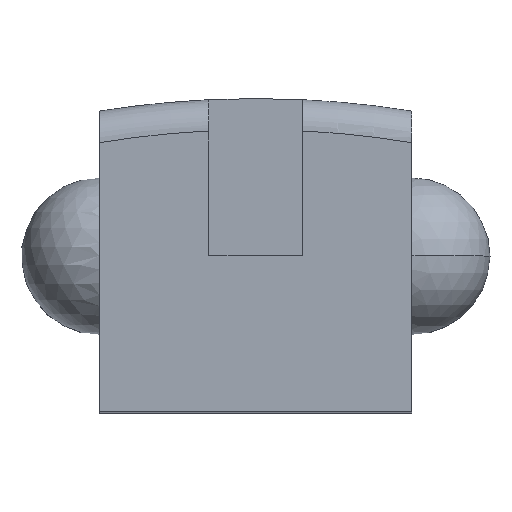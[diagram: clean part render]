
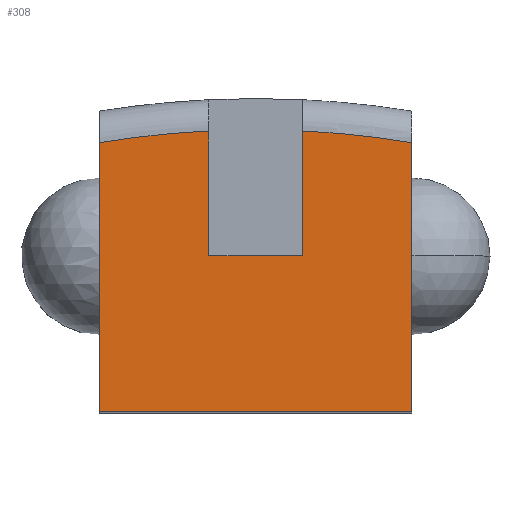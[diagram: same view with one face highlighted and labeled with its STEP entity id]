
A CAD part, top view. The second image highlights one B-rep face of the part: STEP entity #308.
In plain terms, the highlighted planar face has unit normal (0, 0, 1).
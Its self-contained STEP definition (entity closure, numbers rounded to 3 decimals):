
#2 = DIRECTION ( 'NONE',  ( 0., -1., 0. ) ) ;
#4 = CARTESIAN_POINT ( 'NONE',  ( 6.5, -1.25, 12.5 ) ) ;
#25 = CARTESIAN_POINT ( 'NONE',  ( 6.5, -1.25, 12.5 ) ) ;
#34 = DIRECTION ( 'NONE',  ( 0., 0., 1. ) ) ;
#44 = CARTESIAN_POINT ( 'NONE',  ( 3.5, -1.25, 12.5 ) ) ;
#46 = DIRECTION ( 'NONE',  ( 0., 1., 0. ) ) ;
#47 = DIRECTION ( 'NONE',  ( 0., -1., 0. ) ) ;
#55 = DIRECTION ( 'NONE',  ( -1., 0., 0. ) ) ;
#70 = DIRECTION ( 'NONE',  ( 0., 0., 1. ) ) ;
#90 = CARTESIAN_POINT ( 'NONE',  ( 6.5, 2.747, 12.5 ) ) ;
#99 = CARTESIAN_POINT ( 'NONE',  ( 10., -6.25, 12.5 ) ) ;
#117 = CARTESIAN_POINT ( 'NONE',  ( 0., -6.25, 12.5 ) ) ;
#131 = CARTESIAN_POINT ( 'NONE',  ( 10., -6.25, 12.5 ) ) ;
#154 = CARTESIAN_POINT ( 'NONE',  ( 10., 2.371, 12.5 ) ) ;
#155 = CARTESIAN_POINT ( 'NONE',  ( 10., -6.25, 12.5 ) ) ;
#157 = DIRECTION ( 'NONE',  ( 1., 0., 0. ) ) ;
#183 = AXIS2_PLACEMENT_3D ( 'NONE', #237, #34, #309 ) ;
#210 = VECTOR ( 'NONE', #455, 1000. ) ;
#215 = VECTOR ( 'NONE', #233, 1000. ) ;
#217 = LINE ( 'NONE', #155, #210 ) ;
#219 = CIRCLE ( 'NONE', #183, 30.5 ) ;
#220 = LINE ( 'NONE', #99, #215 ) ;
#233 = DIRECTION ( 'NONE',  ( -1., 0., 0. ) ) ;
#237 = CARTESIAN_POINT ( 'NONE',  ( 5., -27.716, 12.5 ) ) ;
#241 = VECTOR ( 'NONE', #2, 1000. ) ;
#249 = LINE ( 'NONE', #303, #241 ) ;
#255 = AXIS2_PLACEMENT_3D ( 'NONE', #293, #70, #55 ) ;
#256 = VECTOR ( 'NONE', #157, 1000. ) ;
#257 = LINE ( 'NONE', #382, #256 ) ;
#260 = CIRCLE ( 'NONE', #255, 30.5 ) ;
#263 = CARTESIAN_POINT ( 'NONE',  ( 3.5, 2.747, 12.5 ) ) ;
#265 = LINE ( 'NONE', #25, #268 ) ;
#268 = VECTOR ( 'NONE', #46, 1000. ) ;
#273 = CARTESIAN_POINT ( 'NONE',  ( 0., -6.25, 12.5 ) ) ;
#275 = DIRECTION ( 'NONE',  ( -1., 0., 0. ) ) ;
#278 = LINE ( 'NONE', #117, #287 ) ;
#281 = DIRECTION ( 'NONE',  ( 0., 0., -1. ) ) ;
#287 = VECTOR ( 'NONE', #47, 1000. ) ;
#292 = FACE_OUTER_BOUND ( 'NONE', #480, .T. ) ;
#293 = CARTESIAN_POINT ( 'NONE',  ( 5., -27.716, 12.5 ) ) ;
#303 = CARTESIAN_POINT ( 'NONE',  ( 3.5, -1.25, 12.5 ) ) ;
#308 = ADVANCED_FACE ( 'NONE', ( #292 ), #311, .F. ) ;
#309 = DIRECTION ( 'NONE',  ( -1., 0., 0. ) ) ;
#311 = PLANE ( 'NONE',  #322 ) ;
#322 = AXIS2_PLACEMENT_3D ( 'NONE', #323, #281, #275 ) ;
#323 = CARTESIAN_POINT ( 'NONE',  ( 10., -6.25, 12.5 ) ) ;
#336 = VERTEX_POINT ( 'NONE', #273 ) ;
#353 = VERTEX_POINT ( 'NONE', #263 ) ;
#360 = CARTESIAN_POINT ( 'NONE',  ( 0., 2.371, 12.5 ) ) ;
#382 = CARTESIAN_POINT ( 'NONE',  ( 3.5, -1.25, 12.5 ) ) ;
#383 = ORIENTED_EDGE ( 'NONE', *, *, #458, .F. ) ;
#387 = VERTEX_POINT ( 'NONE', #154 ) ;
#403 = ORIENTED_EDGE ( 'NONE', *, *, #433, .T. ) ;
#412 = VERTEX_POINT ( 'NONE', #90 ) ;
#433 = EDGE_CURVE ( 'NONE', #527, #336, #278, .T. ) ;
#440 = VERTEX_POINT ( 'NONE', #44 ) ;
#444 = ORIENTED_EDGE ( 'NONE', *, *, #593, .T. ) ;
#445 = EDGE_CURVE ( 'NONE', #569, #412, #265, .T. ) ;
#455 = DIRECTION ( 'NONE',  ( 0., -1., 0. ) ) ;
#458 = EDGE_CURVE ( 'NONE', #440, #569, #257, .T. ) ;
#465 = EDGE_CURVE ( 'NONE', #353, #527, #260, .T. ) ;
#480 = EDGE_LOOP ( 'NONE', ( #383, #583, #504, #403, #600, #518, #444, #613 ) ) ;
#500 = EDGE_CURVE ( 'NONE', #353, #440, #249, .T. ) ;
#504 = ORIENTED_EDGE ( 'NONE', *, *, #465, .T. ) ;
#515 = VERTEX_POINT ( 'NONE', #131 ) ;
#518 = ORIENTED_EDGE ( 'NONE', *, *, #587, .F. ) ;
#527 = VERTEX_POINT ( 'NONE', #360 ) ;
#569 = VERTEX_POINT ( 'NONE', #4 ) ;
#582 = EDGE_CURVE ( 'NONE', #515, #336, #220, .T. ) ;
#583 = ORIENTED_EDGE ( 'NONE', *, *, #500, .F. ) ;
#587 = EDGE_CURVE ( 'NONE', #387, #515, #217, .T. ) ;
#593 = EDGE_CURVE ( 'NONE', #387, #412, #219, .T. ) ;
#600 = ORIENTED_EDGE ( 'NONE', *, *, #582, .F. ) ;
#613 = ORIENTED_EDGE ( 'NONE', *, *, #445, .F. ) ;
